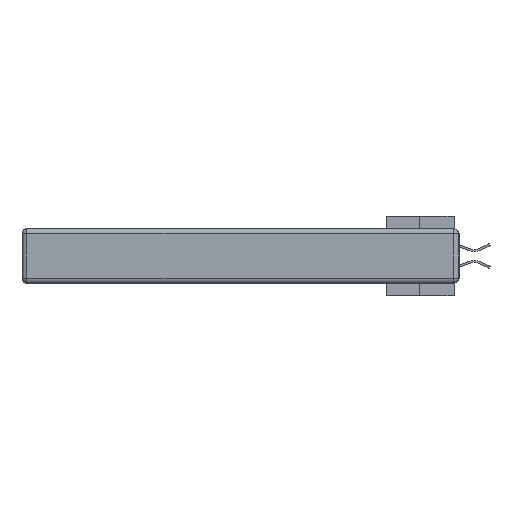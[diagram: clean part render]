
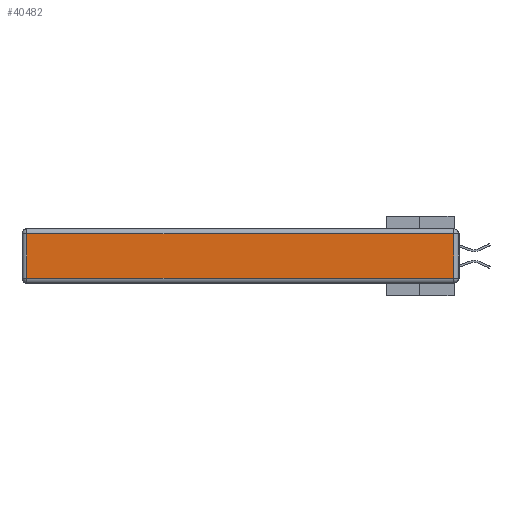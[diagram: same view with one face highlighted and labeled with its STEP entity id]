
A CAD part, left-side view. The second image highlights one B-rep face of the part: STEP entity #40482.
In plain terms, the highlighted planar face has unit normal (-1, 0, 0).
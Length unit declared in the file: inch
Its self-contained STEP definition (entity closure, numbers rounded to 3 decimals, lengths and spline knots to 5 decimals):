
#1682 = VECTOR ( 'NONE', #25356, 39.37008 ) ;
#1805 = VECTOR ( 'NONE', #19126, 39.37008 ) ;
#4062 = VERTEX_POINT ( 'NONE', #27390 ) ;
#5339 = CARTESIAN_POINT ( 'NONE',  ( 0., 0.03, -0.313 ) ) ;
#6162 = VERTEX_POINT ( 'NONE', #18465 ) ;
#9003 = ORIENTED_EDGE ( 'NONE', *, *, #23268, .T. ) ;
#9381 = CARTESIAN_POINT ( 'NONE',  ( 0., 0., -0.313 ) ) ;
#9515 = DIRECTION ( 'NONE',  ( 0., -1., 0. ) ) ;
#9930 = CARTESIAN_POINT ( 'NONE',  ( 0., 2.72, -0.343 ) ) ;
#9932 = VECTOR ( 'NONE', #9515, 39.37008 ) ;
#13752 = CARTESIAN_POINT ( 'NONE',  ( 0., 2.72, -0.03 ) ) ;
#17130 = ORIENTED_EDGE ( 'NONE', *, *, #37589, .T. ) ;
#18465 = CARTESIAN_POINT ( 'NONE',  ( 0., 0.03, -0.03 ) ) ;
#19126 = DIRECTION ( 'NONE',  ( 0., 0., 1. ) ) ;
#19283 = DIRECTION ( 'NONE',  ( 0., 0., 1. ) ) ;
#20409 = LINE ( 'NONE', #9930, #1682 ) ;
#20590 = AXIS2_PLACEMENT_3D ( 'NONE', #31493, #25489, #19283 ) ;
#20766 = ORIENTED_EDGE ( 'NONE', *, *, #33333, .T. ) ;
#22042 = LINE ( 'NONE', #26342, #37739 ) ;
#22181 = ORIENTED_EDGE ( 'NONE', *, *, #40452, .T. ) ;
#23268 = EDGE_CURVE ( 'NONE', #4062, #30494, #24220, .T. ) ;
#23494 = VERTEX_POINT ( 'NONE', #13752 ) ;
#24220 = LINE ( 'NONE', #9381, #9932 ) ;
#25216 = PLANE ( 'NONE',  #20590 ) ;
#25356 = DIRECTION ( 'NONE',  ( 0., 0., -1. ) ) ;
#25489 = DIRECTION ( 'NONE',  ( -1., 0., 0. ) ) ;
#26342 = CARTESIAN_POINT ( 'NONE',  ( 0., 2.75, -0.03 ) ) ;
#27390 = CARTESIAN_POINT ( 'NONE',  ( 0., 2.72, -0.313 ) ) ;
#30494 = VERTEX_POINT ( 'NONE', #5339 ) ;
#31338 = CARTESIAN_POINT ( 'NONE',  ( 0., 0.03, -0.343 ) ) ;
#31493 = CARTESIAN_POINT ( 'NONE',  ( 0., 0., -0.343 ) ) ;
#33333 = EDGE_CURVE ( 'NONE', #6162, #23494, #22042, .T. ) ;
#34192 = EDGE_LOOP ( 'NONE', ( #9003, #17130, #20766, #22181 ) ) ;
#36048 = DIRECTION ( 'NONE',  ( 0., 1., 0. ) ) ;
#36122 = FACE_OUTER_BOUND ( 'NONE', #34192, .T. ) ;
#37210 = LINE ( 'NONE', #31338, #1805 ) ;
#37589 = EDGE_CURVE ( 'NONE', #30494, #6162, #37210, .T. ) ;
#37739 = VECTOR ( 'NONE', #36048, 39.37008 ) ;
#40452 = EDGE_CURVE ( 'NONE', #23494, #4062, #20409, .T. ) ;
#40482 = ADVANCED_FACE ( 'NONE', ( #36122 ), #25216, .T. ) ;
